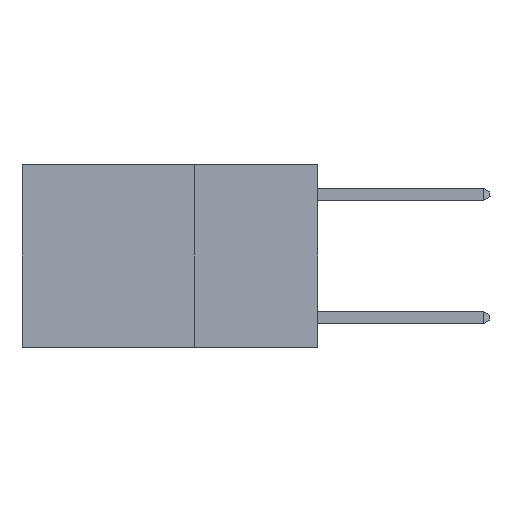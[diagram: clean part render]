
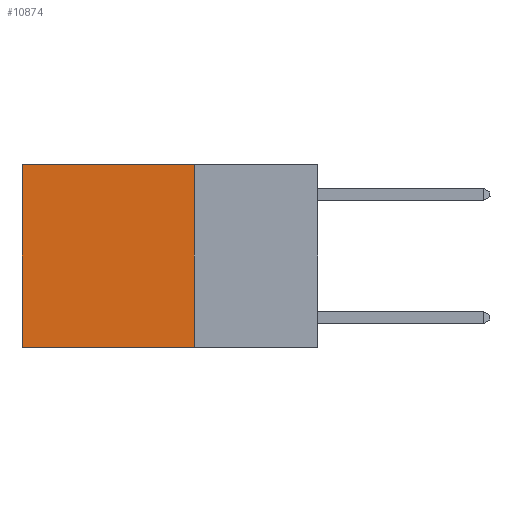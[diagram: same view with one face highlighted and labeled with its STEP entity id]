
A CAD part, left-side view. The second image highlights one B-rep face of the part: STEP entity #10874.
In plain terms, the highlighted planar face has unit normal (-1, 0, 0).
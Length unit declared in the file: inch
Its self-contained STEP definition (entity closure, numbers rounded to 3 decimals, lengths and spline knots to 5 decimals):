
#335 = VERTEX_POINT ( 'NONE', #8832 ) ;
#601 = ORIENTED_EDGE ( 'NONE', *, *, #16398, .T. ) ;
#976 = DIRECTION ( 'NONE',  ( 0., 0., -1. ) ) ;
#1413 = VECTOR ( 'NONE', #976, 39.37008 ) ;
#1585 = VECTOR ( 'NONE', #14484, 39.37008 ) ;
#1774 = LINE ( 'NONE', #13797, #11276 ) ;
#3429 = FACE_OUTER_BOUND ( 'NONE', #11864, .T. ) ;
#3595 = DIRECTION ( 'NONE',  ( 0., 1., 0. ) ) ;
#3925 = EDGE_CURVE ( 'NONE', #11012, #4298, #1774, .T. ) ;
#4298 = VERTEX_POINT ( 'NONE', #5458 ) ;
#5098 = ORIENTED_EDGE ( 'NONE', *, *, #10972, .T. ) ;
#5308 = EDGE_CURVE ( 'NONE', #4298, #335, #12045, .T. ) ;
#5458 = CARTESIAN_POINT ( 'NONE',  ( 0.2625, 0.25, -0.37 ) ) ;
#5623 = ORIENTED_EDGE ( 'NONE', *, *, #3925, .F. ) ;
#6998 = DIRECTION ( 'NONE',  ( 0., 0., -1. ) ) ;
#7590 = ORIENTED_EDGE ( 'NONE', *, *, #5308, .F. ) ;
#8284 = CARTESIAN_POINT ( 'NONE',  ( 0.2625, 0.25, 0. ) ) ;
#8666 = DIRECTION ( 'NONE',  ( 0., 0., -1. ) ) ;
#8832 = CARTESIAN_POINT ( 'NONE',  ( 0.2625, 0.6, -0.37 ) ) ;
#10851 = PLANE ( 'NONE',  #11378 ) ;
#10874 = ADVANCED_FACE ( 'NONE', ( #3429 ), #10851, .F. ) ;
#10972 = EDGE_CURVE ( 'NONE', #16059, #335, #15187, .T. ) ;
#11012 = VERTEX_POINT ( 'NONE', #15215 ) ;
#11276 = VECTOR ( 'NONE', #8666, 39.37008 ) ;
#11360 = CARTESIAN_POINT ( 'NONE',  ( 0.2625, 0.25, -0.37 ) ) ;
#11378 = AXIS2_PLACEMENT_3D ( 'NONE', #8284, #14775, #6998 ) ;
#11864 = EDGE_LOOP ( 'NONE', ( #5098, #7590, #5623, #601 ) ) ;
#12045 = LINE ( 'NONE', #11360, #15907 ) ;
#13196 = CARTESIAN_POINT ( 'NONE',  ( 0.2625, 0.25, 0. ) ) ;
#13797 = CARTESIAN_POINT ( 'NONE',  ( 0.2625, 0.25, 0. ) ) ;
#13816 = CARTESIAN_POINT ( 'NONE',  ( 0.2625, 0.6, 0. ) ) ;
#14484 = DIRECTION ( 'NONE',  ( 0., 1., 0. ) ) ;
#14775 = DIRECTION ( 'NONE',  ( 1., 0., 0. ) ) ;
#15187 = LINE ( 'NONE', #16465, #1413 ) ;
#15215 = CARTESIAN_POINT ( 'NONE',  ( 0.2625, 0.25, 0. ) ) ;
#15346 = LINE ( 'NONE', #13196, #1585 ) ;
#15907 = VECTOR ( 'NONE', #3595, 39.37008 ) ;
#16059 = VERTEX_POINT ( 'NONE', #13816 ) ;
#16398 = EDGE_CURVE ( 'NONE', #11012, #16059, #15346, .T. ) ;
#16465 = CARTESIAN_POINT ( 'NONE',  ( 0.2625, 0.6, 0. ) ) ;
